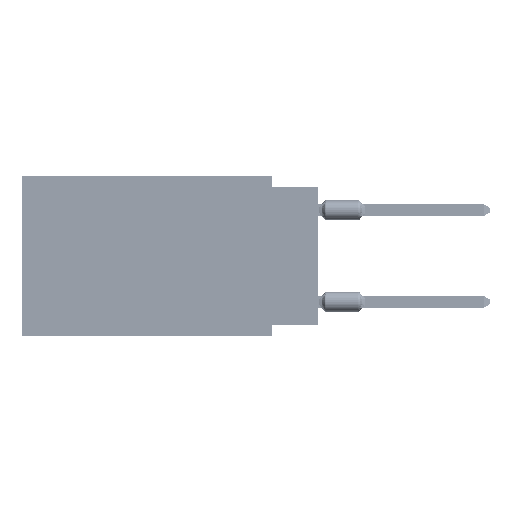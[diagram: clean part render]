
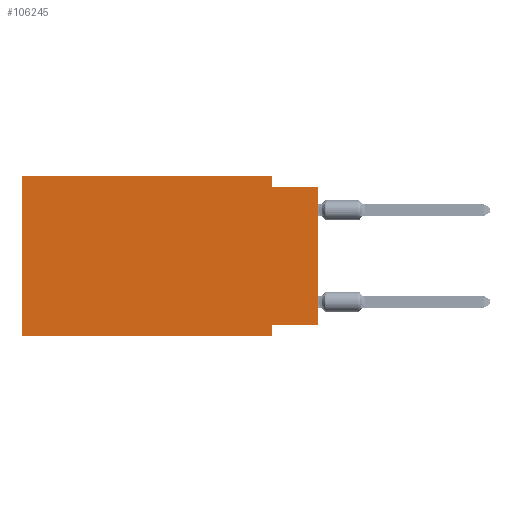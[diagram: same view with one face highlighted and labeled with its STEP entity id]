
A CAD part, left-side view. The second image highlights one B-rep face of the part: STEP entity #106245.
In plain terms, the highlighted planar face has unit normal (-1, 0, 0).
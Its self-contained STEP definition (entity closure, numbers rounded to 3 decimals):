
#1762 = PLANE ( 'NONE',  #29603 ) ;
#1873 = DIRECTION ( 'NONE',  ( 0., 1., 0. ) ) ;
#3041 = ORIENTED_EDGE ( 'NONE', *, *, #28372, .F. ) ;
#4926 = CARTESIAN_POINT ( 'NONE',  ( 0., 2.54, -8.89 ) ) ;
#5736 = LINE ( 'NONE', #48263, #85064 ) ;
#8505 = VECTOR ( 'NONE', #64383, 1000. ) ;
#9398 = CARTESIAN_POINT ( 'NONE',  ( 0., 16.383, 0. ) ) ;
#10285 = VERTEX_POINT ( 'NONE', #20860 ) ;
#12198 = LINE ( 'NONE', #68958, #80153 ) ;
#16515 = DIRECTION ( 'NONE',  ( 1., 0., 0. ) ) ;
#18489 = ORIENTED_EDGE ( 'NONE', *, *, #57263, .F. ) ;
#20623 = DIRECTION ( 'NONE',  ( 0., -1., 0. ) ) ;
#20860 = CARTESIAN_POINT ( 'NONE',  ( 0., 0., -8.255 ) ) ;
#21268 = CARTESIAN_POINT ( 'NONE',  ( 0., 16.383, -8.89 ) ) ;
#26480 = CARTESIAN_POINT ( 'NONE',  ( 0., 2.54, 0. ) ) ;
#27657 = ORIENTED_EDGE ( 'NONE', *, *, #88269, .T. ) ;
#28084 = CARTESIAN_POINT ( 'NONE',  ( 0., 2.54, -0.635 ) ) ;
#28372 = EDGE_CURVE ( 'NONE', #32366, #100495, #56452, .T. ) ;
#29603 = AXIS2_PLACEMENT_3D ( 'NONE', #93401, #16515, #35026 ) ;
#31061 = CARTESIAN_POINT ( 'NONE',  ( 0., 16.383, 0. ) ) ;
#31793 = EDGE_CURVE ( 'NONE', #77901, #64679, #79666, .T. ) ;
#32151 = EDGE_CURVE ( 'NONE', #100495, #67154, #102494, .T. ) ;
#32366 = VERTEX_POINT ( 'NONE', #26480 ) ;
#35026 = DIRECTION ( 'NONE',  ( 0., 0., -1. ) ) ;
#36001 = CARTESIAN_POINT ( 'NONE',  ( 0., 2.54, -8.255 ) ) ;
#41705 = CARTESIAN_POINT ( 'NONE',  ( 0., 16.383, -8.89 ) ) ;
#43190 = LINE ( 'NONE', #9398, #76570 ) ;
#48263 = CARTESIAN_POINT ( 'NONE',  ( 0., 16.383, 0. ) ) ;
#48811 = EDGE_CURVE ( 'NONE', #10285, #77901, #12198, .T. ) ;
#51542 = VECTOR ( 'NONE', #57539, 1000. ) ;
#55359 = DIRECTION ( 'NONE',  ( 0., -1., 0. ) ) ;
#56452 = LINE ( 'NONE', #65192, #51542 ) ;
#57263 = EDGE_CURVE ( 'NONE', #70000, #70047, #43190, .T. ) ;
#57539 = DIRECTION ( 'NONE',  ( 0., 0., -1. ) ) ;
#59044 = VECTOR ( 'NONE', #20623, 1000. ) ;
#64383 = DIRECTION ( 'NONE',  ( 0., 0., -1. ) ) ;
#64679 = VERTEX_POINT ( 'NONE', #99728 ) ;
#64735 = EDGE_LOOP ( 'NONE', ( #27657, #96303, #3041, #83153, #18489, #77363, #101832, #104343 ) ) ;
#65192 = CARTESIAN_POINT ( 'NONE',  ( 0., 2.54, 0. ) ) ;
#65748 = LINE ( 'NONE', #41705, #66945 ) ;
#66945 = VECTOR ( 'NONE', #99035, 1000. ) ;
#67154 = VERTEX_POINT ( 'NONE', #90632 ) ;
#68958 = CARTESIAN_POINT ( 'NONE',  ( 0., 0., -8.255 ) ) ;
#70000 = VERTEX_POINT ( 'NONE', #21268 ) ;
#70047 = VERTEX_POINT ( 'NONE', #31061 ) ;
#76480 = FACE_OUTER_BOUND ( 'NONE', #64735, .T. ) ;
#76570 = VECTOR ( 'NONE', #102117, 1000. ) ;
#77363 = ORIENTED_EDGE ( 'NONE', *, *, #88796, .T. ) ;
#77376 = VECTOR ( 'NONE', #78061, 1000. ) ;
#77901 = VERTEX_POINT ( 'NONE', #36001 ) ;
#78061 = DIRECTION ( 'NONE',  ( 0., 0., 1. ) ) ;
#79666 = LINE ( 'NONE', #4926, #8505 ) ;
#80153 = VECTOR ( 'NONE', #1873, 1000. ) ;
#83153 = ORIENTED_EDGE ( 'NONE', *, *, #102800, .F. ) ;
#85064 = VECTOR ( 'NONE', #55359, 1000. ) ;
#86259 = LINE ( 'NONE', #86794, #77376 ) ;
#86794 = CARTESIAN_POINT ( 'NONE',  ( 0., 0., 0. ) ) ;
#88269 = EDGE_CURVE ( 'NONE', #10285, #67154, #86259, .T. ) ;
#88796 = EDGE_CURVE ( 'NONE', #70000, #64679, #65748, .T. ) ;
#90632 = CARTESIAN_POINT ( 'NONE',  ( 0., 0., -0.635 ) ) ;
#93223 = CARTESIAN_POINT ( 'NONE',  ( 0., 0., -0.635 ) ) ;
#93401 = CARTESIAN_POINT ( 'NONE',  ( 0., 16.383, 0. ) ) ;
#96303 = ORIENTED_EDGE ( 'NONE', *, *, #32151, .F. ) ;
#99035 = DIRECTION ( 'NONE',  ( 0., -1., 0. ) ) ;
#99728 = CARTESIAN_POINT ( 'NONE',  ( 0., 2.54, -8.89 ) ) ;
#100495 = VERTEX_POINT ( 'NONE', #28084 ) ;
#101832 = ORIENTED_EDGE ( 'NONE', *, *, #31793, .F. ) ;
#102117 = DIRECTION ( 'NONE',  ( 0., 0., 1. ) ) ;
#102494 = LINE ( 'NONE', #93223, #59044 ) ;
#102800 = EDGE_CURVE ( 'NONE', #70047, #32366, #5736, .T. ) ;
#104343 = ORIENTED_EDGE ( 'NONE', *, *, #48811, .F. ) ;
#106245 = ADVANCED_FACE ( 'NONE', ( #76480 ), #1762, .F. ) ;
